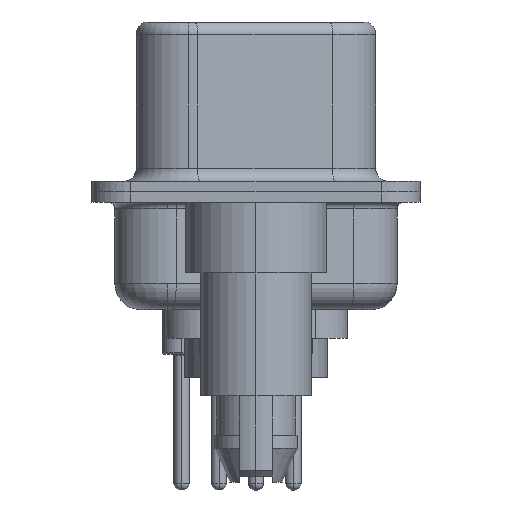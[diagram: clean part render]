
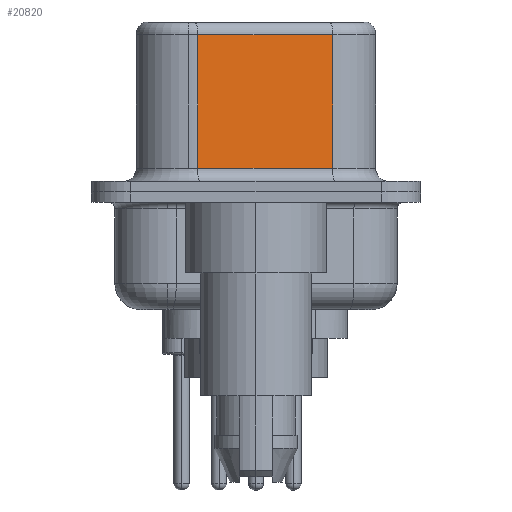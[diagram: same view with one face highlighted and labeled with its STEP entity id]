
A CAD part, left-side view. The second image highlights one B-rep face of the part: STEP entity #20820.
In plain terms, the highlighted planar face has unit normal (-0.985, -0.174, 0).
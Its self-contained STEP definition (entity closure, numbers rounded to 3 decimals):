
#470 = VERTEX_POINT ( 'NONE', #15301 ) ;
#914 = FACE_OUTER_BOUND ( 'NONE', #16928, .T. ) ;
#1065 = CARTESIAN_POINT ( 'NONE',  ( 4.585, -2.927, 6.52 ) ) ;
#1322 = VECTOR ( 'NONE', #6400, 1000. ) ;
#2406 = LINE ( 'NONE', #1065, #14603 ) ;
#2896 = LINE ( 'NONE', #16350, #1322 ) ;
#3015 = CARTESIAN_POINT ( 'NONE',  ( 4.585, -2.927, 6.52 ) ) ;
#3489 = DIRECTION ( 'NONE',  ( 0.174, -0.985, 0. ) ) ;
#3639 = CARTESIAN_POINT ( 'NONE',  ( 3.675, 2.233, 0.9 ) ) ;
#3910 = CARTESIAN_POINT ( 'NONE',  ( 3.675, 2.233, 6.52 ) ) ;
#5361 = DIRECTION ( 'NONE',  ( 0., 0., -1. ) ) ;
#6400 = DIRECTION ( 'NONE',  ( -0.174, 0.985, 0. ) ) ;
#8175 = EDGE_CURVE ( 'NONE', #12820, #10404, #2896, .T. ) ;
#8184 = LINE ( 'NONE', #13356, #17845 ) ;
#9425 = PLANE ( 'NONE',  #15058 ) ;
#9474 = ORIENTED_EDGE ( 'NONE', *, *, #9937, .T. ) ;
#9937 = EDGE_CURVE ( 'NONE', #10404, #10115, #11894, .T. ) ;
#10115 = VERTEX_POINT ( 'NONE', #3639 ) ;
#10317 = VECTOR ( 'NONE', #5361, 1000. ) ;
#10404 = VERTEX_POINT ( 'NONE', #15175 ) ;
#11894 = LINE ( 'NONE', #3910, #10317 ) ;
#12159 = EDGE_CURVE ( 'NONE', #10115, #470, #8184, .T. ) ;
#12820 = VERTEX_POINT ( 'NONE', #20494 ) ;
#13356 = CARTESIAN_POINT ( 'NONE',  ( 4.585, -2.927, 0.9 ) ) ;
#14190 = ORIENTED_EDGE ( 'NONE', *, *, #15784, .F. ) ;
#14603 = VECTOR ( 'NONE', #19174, 1000. ) ;
#15058 = AXIS2_PLACEMENT_3D ( 'NONE', #3015, #17997, #21114 ) ;
#15175 = CARTESIAN_POINT ( 'NONE',  ( 3.675, 2.233, 6.02 ) ) ;
#15301 = CARTESIAN_POINT ( 'NONE',  ( 4.585, -2.927, 0.9 ) ) ;
#15784 = EDGE_CURVE ( 'NONE', #12820, #470, #2406, .T. ) ;
#16119 = ORIENTED_EDGE ( 'NONE', *, *, #12159, .T. ) ;
#16350 = CARTESIAN_POINT ( 'NONE',  ( 4.585, -2.927, 6.02 ) ) ;
#16928 = EDGE_LOOP ( 'NONE', ( #14190, #20971, #9474, #16119 ) ) ;
#17845 = VECTOR ( 'NONE', #3489, 1000. ) ;
#17997 = DIRECTION ( 'NONE',  ( 0.985, 0.174, 0. ) ) ;
#19174 = DIRECTION ( 'NONE',  ( 0., 0., -1. ) ) ;
#20494 = CARTESIAN_POINT ( 'NONE',  ( 4.585, -2.927, 6.02 ) ) ;
#20820 = ADVANCED_FACE ( 'NONE', ( #914 ), #9425, .F. ) ;
#20971 = ORIENTED_EDGE ( 'NONE', *, *, #8175, .T. ) ;
#21114 = DIRECTION ( 'NONE',  ( -0.174, 0.985, 0. ) ) ;
